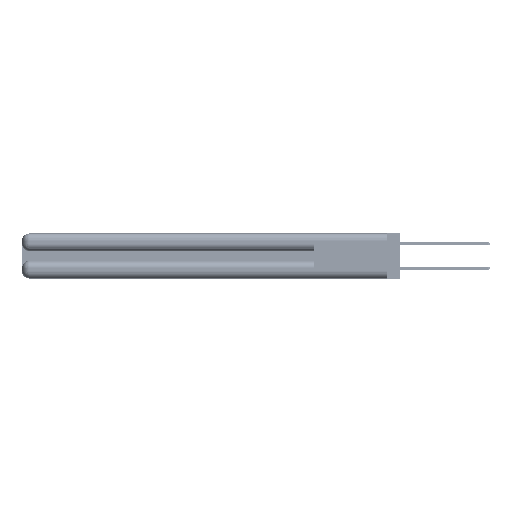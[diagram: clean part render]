
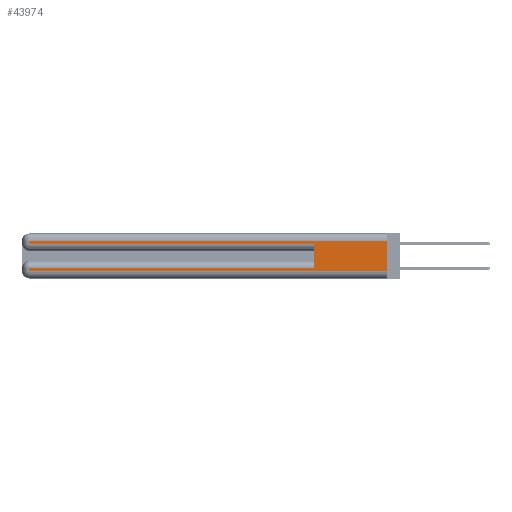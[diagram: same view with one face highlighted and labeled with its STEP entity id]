
A CAD part, left-side view. The second image highlights one B-rep face of the part: STEP entity #43974.
In plain terms, the highlighted planar face has unit normal (-1, 0, 0).
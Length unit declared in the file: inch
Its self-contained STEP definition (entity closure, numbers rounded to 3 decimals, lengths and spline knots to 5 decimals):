
#74 = DIRECTION ( 'NONE',  ( 0., 0., -1. ) ) ;
#838 = VECTOR ( 'NONE', #8342, 39.37008 ) ;
#1482 = LINE ( 'NONE', #40767, #46445 ) ;
#1595 = VERTEX_POINT ( 'NONE', #27468 ) ;
#2196 = ORIENTED_EDGE ( 'NONE', *, *, #16551, .T. ) ;
#3479 = CARTESIAN_POINT ( 'NONE',  ( 0., 0., 0.31 ) ) ;
#5333 = AXIS2_PLACEMENT_3D ( 'NONE', #34703, #26146, #74 ) ;
#6296 = LINE ( 'NONE', #34316, #51223 ) ;
#7177 = VERTEX_POINT ( 'NONE', #37646 ) ;
#8235 = ORIENTED_EDGE ( 'NONE', *, *, #41366, .T. ) ;
#8342 = DIRECTION ( 'NONE',  ( 0., 0., -1. ) ) ;
#8460 = CARTESIAN_POINT ( 'NONE',  ( 0., 0., 0.37 ) ) ;
#10717 = LINE ( 'NONE', #25024, #32518 ) ;
#10745 = VECTOR ( 'NONE', #21200, 39.37008 ) ;
#11031 = CARTESIAN_POINT ( 'NONE',  ( 0., 0.6, 0.285 ) ) ;
#16404 = ORIENTED_EDGE ( 'NONE', *, *, #35852, .T. ) ;
#16551 = EDGE_CURVE ( 'NONE', #25813, #56306, #45883, .T. ) ;
#16781 = CARTESIAN_POINT ( 'NONE',  ( 0., 2.94, 0.37 ) ) ;
#17156 = VERTEX_POINT ( 'NONE', #29702 ) ;
#19798 = EDGE_CURVE ( 'NONE', #49902, #53213, #10717, .T. ) ;
#19886 = EDGE_CURVE ( 'NONE', #25813, #17156, #38658, .T. ) ;
#21200 = DIRECTION ( 'NONE',  ( 0., 0., -1. ) ) ;
#24379 = CARTESIAN_POINT ( 'NONE',  ( 0., 2.94, 0.085 ) ) ;
#25024 = CARTESIAN_POINT ( 'NONE',  ( 0., 0.6, 0.145 ) ) ;
#25329 = CARTESIAN_POINT ( 'NONE',  ( 0., 0.6, 0.085 ) ) ;
#25813 = VERTEX_POINT ( 'NONE', #37722 ) ;
#26146 = DIRECTION ( 'NONE',  ( 1., 0., 0. ) ) ;
#26819 = DIRECTION ( 'NONE',  ( 0., -1., 0. ) ) ;
#27468 = CARTESIAN_POINT ( 'NONE',  ( 0., 2.94, 0.285 ) ) ;
#27621 = DIRECTION ( 'NONE',  ( 0., 1., 0. ) ) ;
#28011 = ORIENTED_EDGE ( 'NONE', *, *, #41030, .T. ) ;
#29702 = CARTESIAN_POINT ( 'NONE',  ( 0., 0., 0.06 ) ) ;
#30119 = VECTOR ( 'NONE', #26819, 39.37008 ) ;
#31001 = EDGE_LOOP ( 'NONE', ( #52145, #2196, #53371, #28011, #36990, #8235, #16404, #32271 ) ) ;
#31482 = LINE ( 'NONE', #39795, #30119 ) ;
#32271 = ORIENTED_EDGE ( 'NONE', *, *, #48300, .T. ) ;
#32518 = VECTOR ( 'NONE', #33774, 39.37008 ) ;
#33242 = FACE_OUTER_BOUND ( 'NONE', #31001, .T. ) ;
#33774 = DIRECTION ( 'NONE',  ( 0., 0., 1. ) ) ;
#33917 = CARTESIAN_POINT ( 'NONE',  ( 0., 2.94, 0.31 ) ) ;
#34269 = VECTOR ( 'NONE', #51435, 39.37008 ) ;
#34316 = CARTESIAN_POINT ( 'NONE',  ( 0., 0., 0.285 ) ) ;
#34703 = CARTESIAN_POINT ( 'NONE',  ( 0., 0., 0.37 ) ) ;
#35852 = EDGE_CURVE ( 'NONE', #39853, #7177, #47168, .T. ) ;
#36990 = ORIENTED_EDGE ( 'NONE', *, *, #19798, .F. ) ;
#37646 = CARTESIAN_POINT ( 'NONE',  ( 0., 2.94, 0.06 ) ) ;
#37722 = CARTESIAN_POINT ( 'NONE',  ( 0., 0., 0.31 ) ) ;
#38622 = CARTESIAN_POINT ( 'NONE',  ( 0., 2.94, 0.37 ) ) ;
#38658 = LINE ( 'NONE', #8460, #40028 ) ;
#38926 = DIRECTION ( 'NONE',  ( 0., 0., -1. ) ) ;
#39795 = CARTESIAN_POINT ( 'NONE',  ( 0., 0., 0.06 ) ) ;
#39853 = VERTEX_POINT ( 'NONE', #24379 ) ;
#40028 = VECTOR ( 'NONE', #38926, 39.37008 ) ;
#40767 = CARTESIAN_POINT ( 'NONE',  ( 0., 0., 0.085 ) ) ;
#41030 = EDGE_CURVE ( 'NONE', #1595, #53213, #6296, .T. ) ;
#41366 = EDGE_CURVE ( 'NONE', #49902, #39853, #1482, .T. ) ;
#43974 = ADVANCED_FACE ( 'NONE', ( #33242 ), #52213, .F. ) ;
#45548 = LINE ( 'NONE', #16781, #10745 ) ;
#45883 = LINE ( 'NONE', #3479, #34269 ) ;
#46445 = VECTOR ( 'NONE', #27621, 39.37008 ) ;
#47168 = LINE ( 'NONE', #38622, #838 ) ;
#48300 = EDGE_CURVE ( 'NONE', #7177, #17156, #31482, .T. ) ;
#49902 = VERTEX_POINT ( 'NONE', #25329 ) ;
#51223 = VECTOR ( 'NONE', #51820, 39.37008 ) ;
#51265 = EDGE_CURVE ( 'NONE', #56306, #1595, #45548, .T. ) ;
#51435 = DIRECTION ( 'NONE',  ( 0., 1., 0. ) ) ;
#51820 = DIRECTION ( 'NONE',  ( 0., -1., 0. ) ) ;
#52145 = ORIENTED_EDGE ( 'NONE', *, *, #19886, .F. ) ;
#52213 = PLANE ( 'NONE',  #5333 ) ;
#53213 = VERTEX_POINT ( 'NONE', #11031 ) ;
#53371 = ORIENTED_EDGE ( 'NONE', *, *, #51265, .T. ) ;
#56306 = VERTEX_POINT ( 'NONE', #33917 ) ;
